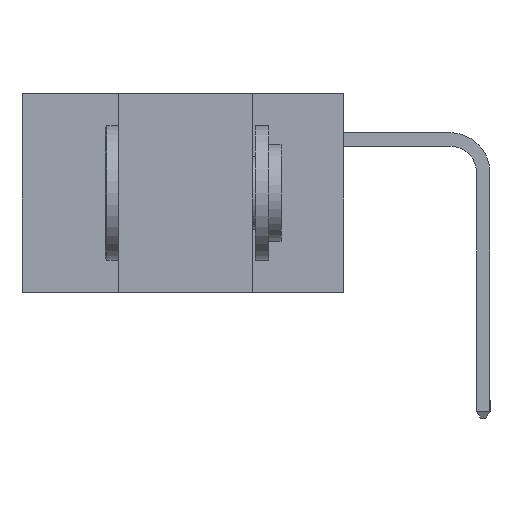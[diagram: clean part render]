
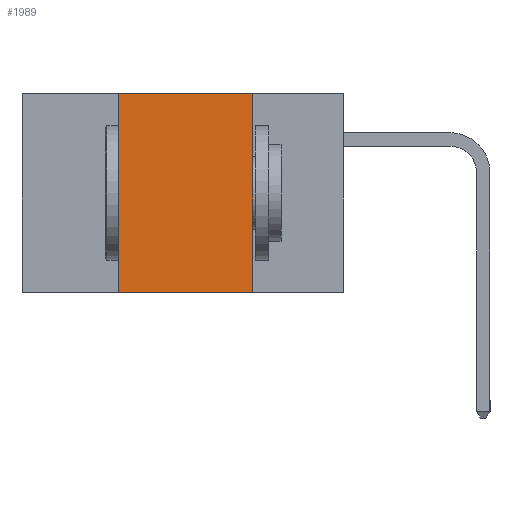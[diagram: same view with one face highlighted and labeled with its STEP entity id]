
A CAD part, left-side view. The second image highlights one B-rep face of the part: STEP entity #1989.
In plain terms, the highlighted planar face has unit normal (-1, 0, 0).
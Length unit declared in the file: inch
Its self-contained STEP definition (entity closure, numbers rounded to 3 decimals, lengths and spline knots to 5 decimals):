
#112 = CARTESIAN_POINT ( 'NONE',  ( 0., 0.6, 0. ) ) ;
#601 = LINE ( 'NONE', #15191, #20920 ) ;
#1564 = PLANE ( 'NONE',  #10436 ) ;
#1989 = ADVANCED_FACE ( 'NONE', ( #16687 ), #1564, .F. ) ;
#2586 = EDGE_CURVE ( 'NONE', #18640, #14574, #12571, .T. ) ;
#2925 = EDGE_CURVE ( 'NONE', #22701, #22171, #20459, .T. ) ;
#3701 = DIRECTION ( 'NONE',  ( 0., 0., -1. ) ) ;
#4495 = CARTESIAN_POINT ( 'NONE',  ( 0., 0.42, -0.37 ) ) ;
#5351 = VECTOR ( 'NONE', #9011, 39.37008 ) ;
#7359 = EDGE_CURVE ( 'NONE', #18640, #22701, #17430, .T. ) ;
#7481 = VECTOR ( 'NONE', #23191, 39.37008 ) ;
#7986 = DIRECTION ( 'NONE',  ( 1., 0., 0. ) ) ;
#8395 = CARTESIAN_POINT ( 'NONE',  ( 0., 0.6, 0. ) ) ;
#8473 = ORIENTED_EDGE ( 'NONE', *, *, #2925, .F. ) ;
#9011 = DIRECTION ( 'NONE',  ( 0., -1., 0. ) ) ;
#10277 = ORIENTED_EDGE ( 'NONE', *, *, #2586, .T. ) ;
#10379 = EDGE_LOOP ( 'NONE', ( #21386, #8473, #18487, #10277 ) ) ;
#10436 = AXIS2_PLACEMENT_3D ( 'NONE', #112, #7986, #14139 ) ;
#12571 = LINE ( 'NONE', #20633, #7481 ) ;
#14139 = DIRECTION ( 'NONE',  ( 0., 0., -1. ) ) ;
#14574 = VERTEX_POINT ( 'NONE', #18348 ) ;
#15191 = CARTESIAN_POINT ( 'NONE',  ( 0., 0.17, -0.37 ) ) ;
#16687 = FACE_OUTER_BOUND ( 'NONE', #10379, .T. ) ;
#17430 = LINE ( 'NONE', #21046, #22343 ) ;
#18348 = CARTESIAN_POINT ( 'NONE',  ( 0., 0.17, -0.37 ) ) ;
#18487 = ORIENTED_EDGE ( 'NONE', *, *, #7359, .F. ) ;
#18640 = VERTEX_POINT ( 'NONE', #4495 ) ;
#19547 = EDGE_CURVE ( 'NONE', #22171, #14574, #601, .T. ) ;
#20259 = CARTESIAN_POINT ( 'NONE',  ( 0., 0.42, 0. ) ) ;
#20459 = LINE ( 'NONE', #8395, #5351 ) ;
#20633 = CARTESIAN_POINT ( 'NONE',  ( 0., 0.6, -0.37 ) ) ;
#20778 = DIRECTION ( 'NONE',  ( 0., 0., 1. ) ) ;
#20920 = VECTOR ( 'NONE', #3701, 39.37008 ) ;
#21046 = CARTESIAN_POINT ( 'NONE',  ( 0., 0.42, -0.37 ) ) ;
#21386 = ORIENTED_EDGE ( 'NONE', *, *, #19547, .F. ) ;
#22171 = VERTEX_POINT ( 'NONE', #24159 ) ;
#22343 = VECTOR ( 'NONE', #20778, 39.37008 ) ;
#22701 = VERTEX_POINT ( 'NONE', #20259 ) ;
#23191 = DIRECTION ( 'NONE',  ( 0., -1., 0. ) ) ;
#24159 = CARTESIAN_POINT ( 'NONE',  ( 0., 0.17, 0. ) ) ;
